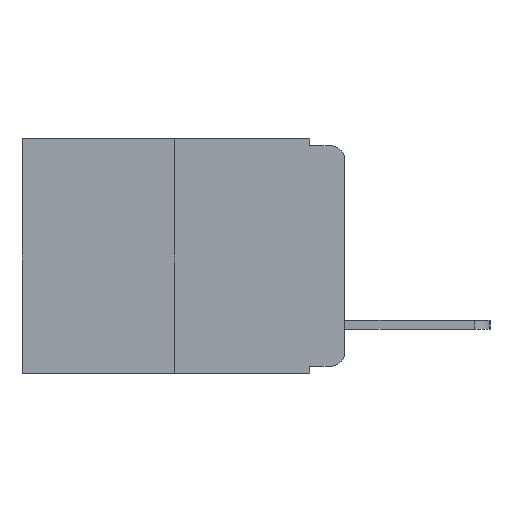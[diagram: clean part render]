
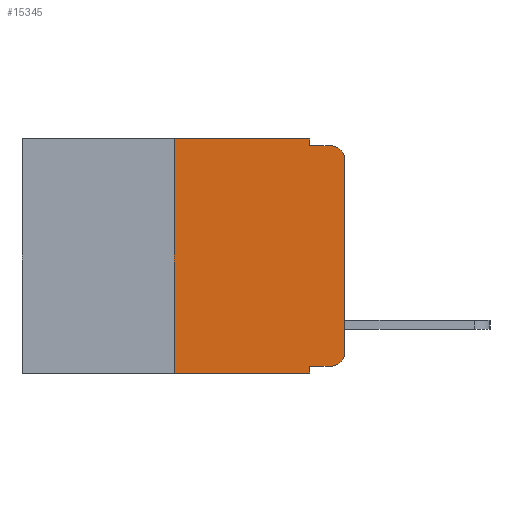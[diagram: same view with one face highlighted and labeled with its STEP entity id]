
A CAD part, left-side view. The second image highlights one B-rep face of the part: STEP entity #15345.
In plain terms, the highlighted planar face has unit normal (-1, 0, 0).
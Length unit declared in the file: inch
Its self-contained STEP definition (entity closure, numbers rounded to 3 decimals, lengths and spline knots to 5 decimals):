
#145 = ORIENTED_EDGE ( 'NONE', *, *, #4958, .T. ) ;
#316 = CARTESIAN_POINT ( 'NONE',  ( 0., 0.25, 0. ) ) ;
#467 = CIRCLE ( 'NONE', #10945, 0.02 ) ;
#722 = LINE ( 'NONE', #12526, #14115 ) ;
#837 = LINE ( 'NONE', #5617, #6613 ) ;
#995 = DIRECTION ( 'NONE',  ( 0., 0., 1. ) ) ;
#1017 = DIRECTION ( 'NONE',  ( 0., -1., 0. ) ) ;
#1155 = LINE ( 'NONE', #6616, #13161 ) ;
#1927 = DIRECTION ( 'NONE',  ( 0., 0., -1. ) ) ;
#2073 = CARTESIAN_POINT ( 'NONE',  ( 0., 0.02, -0.333 ) ) ;
#2087 = CARTESIAN_POINT ( 'NONE',  ( 0., 0.051, 0. ) ) ;
#2222 = DIRECTION ( 'NONE',  ( 0., 0., -1. ) ) ;
#2241 = CARTESIAN_POINT ( 'NONE',  ( 0., 0.02, -0.313 ) ) ;
#2410 = CARTESIAN_POINT ( 'NONE',  ( 0., 0.051, -0.343 ) ) ;
#2488 = CARTESIAN_POINT ( 'NONE',  ( 0., 0.051, -0.01 ) ) ;
#2584 = VERTEX_POINT ( 'NONE', #3923 ) ;
#2788 = VERTEX_POINT ( 'NONE', #2410 ) ;
#2879 = CARTESIAN_POINT ( 'NONE',  ( 0., 0.473, 0. ) ) ;
#3156 = DIRECTION ( 'NONE',  ( 1., 0., 0. ) ) ;
#3227 = VECTOR ( 'NONE', #12632, 39.37008 ) ;
#3233 = DIRECTION ( 'NONE',  ( 0., 0., -1. ) ) ;
#3253 = ORIENTED_EDGE ( 'NONE', *, *, #12746, .T. ) ;
#3442 = EDGE_CURVE ( 'NONE', #6406, #6800, #5656, .T. ) ;
#3923 = CARTESIAN_POINT ( 'NONE',  ( 0., 0.25, -0.343 ) ) ;
#4090 = AXIS2_PLACEMENT_3D ( 'NONE', #8901, #11016, #1927 ) ;
#4215 = EDGE_CURVE ( 'NONE', #5138, #6526, #13576, .T. ) ;
#4654 = ORIENTED_EDGE ( 'NONE', *, *, #3442, .F. ) ;
#4768 = VERTEX_POINT ( 'NONE', #2073 ) ;
#4890 = CARTESIAN_POINT ( 'NONE',  ( 0., 0.25, 0. ) ) ;
#4910 = ORIENTED_EDGE ( 'NONE', *, *, #4215, .F. ) ;
#4958 = EDGE_CURVE ( 'NONE', #8978, #8828, #1155, .T. ) ;
#5058 = DIRECTION ( 'NONE',  ( 0., -1., 0. ) ) ;
#5138 = VERTEX_POINT ( 'NONE', #4890 ) ;
#5253 = ORIENTED_EDGE ( 'NONE', *, *, #6174, .T. ) ;
#5617 = CARTESIAN_POINT ( 'NONE',  ( 0., 0.473, -0.343 ) ) ;
#5634 = DIRECTION ( 'NONE',  ( 0., 0., -1. ) ) ;
#5656 = LINE ( 'NONE', #7003, #13742 ) ;
#5837 = ORIENTED_EDGE ( 'NONE', *, *, #6146, .T. ) ;
#5865 = CARTESIAN_POINT ( 'NONE',  ( 0., 0.051, -0.333 ) ) ;
#6146 = EDGE_CURVE ( 'NONE', #4768, #8978, #467, .T. ) ;
#6174 = EDGE_CURVE ( 'NONE', #8883, #4768, #12800, .T. ) ;
#6406 = VERTEX_POINT ( 'NONE', #2488 ) ;
#6526 = VERTEX_POINT ( 'NONE', #2087 ) ;
#6613 = VECTOR ( 'NONE', #5058, 39.37008 ) ;
#6616 = CARTESIAN_POINT ( 'NONE',  ( 0., 0., 0. ) ) ;
#6734 = CARTESIAN_POINT ( 'NONE',  ( 0., 0.051, 0. ) ) ;
#6800 = VERTEX_POINT ( 'NONE', #14404 ) ;
#6857 = CARTESIAN_POINT ( 'NONE',  ( 0., 0., -0.03 ) ) ;
#7003 = CARTESIAN_POINT ( 'NONE',  ( 0., 0.051, -0.01 ) ) ;
#7063 = VECTOR ( 'NONE', #2222, 39.37008 ) ;
#7218 = LINE ( 'NONE', #316, #12764 ) ;
#7640 = EDGE_LOOP ( 'NONE', ( #145, #3253, #4654, #13780, #4910, #14615, #10786, #13877, #5253, #5837 ) ) ;
#7867 = EDGE_CURVE ( 'NONE', #8883, #2788, #9208, .T. ) ;
#8828 = VERTEX_POINT ( 'NONE', #6857 ) ;
#8883 = VERTEX_POINT ( 'NONE', #14147 ) ;
#8901 = CARTESIAN_POINT ( 'NONE',  ( 0., 0.02, -0.03 ) ) ;
#8978 = VERTEX_POINT ( 'NONE', #13888 ) ;
#9208 = LINE ( 'NONE', #6734, #7063 ) ;
#9660 = EDGE_CURVE ( 'NONE', #2584, #5138, #7218, .T. ) ;
#10269 = PLANE ( 'NONE',  #10386 ) ;
#10386 = AXIS2_PLACEMENT_3D ( 'NONE', #15014, #3156, #3233 ) ;
#10786 = ORIENTED_EDGE ( 'NONE', *, *, #12947, .T. ) ;
#10945 = AXIS2_PLACEMENT_3D ( 'NONE', #2241, #11552, #5634 ) ;
#11016 = DIRECTION ( 'NONE',  ( -1., 0., 0. ) ) ;
#11354 = DIRECTION ( 'NONE',  ( 0., 0., -1. ) ) ;
#11552 = DIRECTION ( 'NONE',  ( -1., 0., 0. ) ) ;
#12054 = CIRCLE ( 'NONE', #4090, 0.02 ) ;
#12526 = CARTESIAN_POINT ( 'NONE',  ( 0., 0.051, 0. ) ) ;
#12632 = DIRECTION ( 'NONE',  ( 0., -1., 0. ) ) ;
#12746 = EDGE_CURVE ( 'NONE', #8828, #6800, #12054, .T. ) ;
#12764 = VECTOR ( 'NONE', #15454, 39.37008 ) ;
#12800 = LINE ( 'NONE', #5865, #13439 ) ;
#12947 = EDGE_CURVE ( 'NONE', #2584, #2788, #837, .T. ) ;
#13161 = VECTOR ( 'NONE', #995, 39.37008 ) ;
#13439 = VECTOR ( 'NONE', #14979, 39.37008 ) ;
#13576 = LINE ( 'NONE', #2879, #3227 ) ;
#13742 = VECTOR ( 'NONE', #1017, 39.37008 ) ;
#13780 = ORIENTED_EDGE ( 'NONE', *, *, #15338, .F. ) ;
#13877 = ORIENTED_EDGE ( 'NONE', *, *, #7867, .F. ) ;
#13888 = CARTESIAN_POINT ( 'NONE',  ( 0., 0., -0.313 ) ) ;
#13924 = FACE_OUTER_BOUND ( 'NONE', #7640, .T. ) ;
#14115 = VECTOR ( 'NONE', #11354, 39.37008 ) ;
#14147 = CARTESIAN_POINT ( 'NONE',  ( 0., 0.051, -0.333 ) ) ;
#14404 = CARTESIAN_POINT ( 'NONE',  ( 0., 0.02, -0.01 ) ) ;
#14615 = ORIENTED_EDGE ( 'NONE', *, *, #9660, .F. ) ;
#14979 = DIRECTION ( 'NONE',  ( 0., -1., 0. ) ) ;
#15014 = CARTESIAN_POINT ( 'NONE',  ( 0., 0.473, 0. ) ) ;
#15338 = EDGE_CURVE ( 'NONE', #6526, #6406, #722, .T. ) ;
#15345 = ADVANCED_FACE ( 'NONE', ( #13924 ), #10269, .F. ) ;
#15454 = DIRECTION ( 'NONE',  ( 0., 0., 1. ) ) ;
